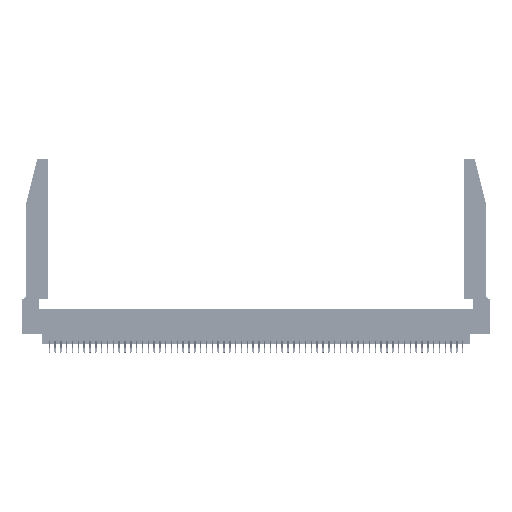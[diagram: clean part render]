
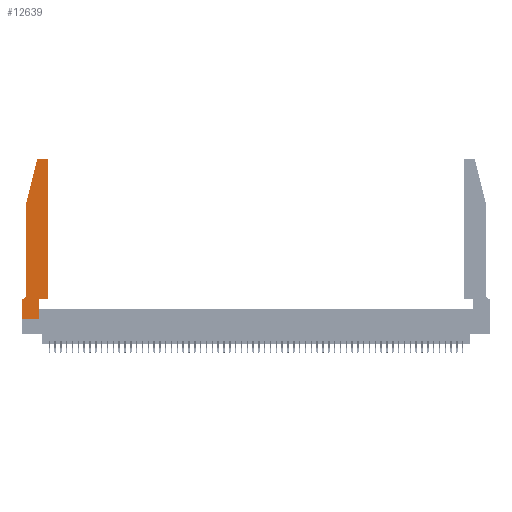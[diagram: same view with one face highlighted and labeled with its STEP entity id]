
A CAD part, top view. The second image highlights one B-rep face of the part: STEP entity #12639.
In plain terms, the highlighted planar face has unit normal (0, 0, 1).
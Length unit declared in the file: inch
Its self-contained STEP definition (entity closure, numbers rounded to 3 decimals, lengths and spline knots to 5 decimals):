
#2148 = CARTESIAN_POINT ( 'NONE',  ( 0.0055, 0.35, 0.37 ) ) ;
#2251 = LINE ( 'NONE', #49824, #40567 ) ;
#2610 = DIRECTION ( 'NONE',  ( -1., 0., 0. ) ) ;
#2852 = VECTOR ( 'NONE', #40689, 39.37008 ) ;
#3091 = ORIENTED_EDGE ( 'NONE', *, *, #7677, .T. ) ;
#3699 = CARTESIAN_POINT ( 'NONE',  ( 0.4505, 2.72, 0.37 ) ) ;
#4174 = CARTESIAN_POINT ( 'NONE',  ( 0.2865, 0., 0.37 ) ) ;
#4948 = EDGE_CURVE ( 'NONE', #49151, #29414, #12987, .T. ) ;
#5057 = CARTESIAN_POINT ( 'NONE',  ( 0., 0., 0.37 ) ) ;
#5948 = CARTESIAN_POINT ( 'NONE',  ( 0.4505, 0.35, 0.37 ) ) ;
#7371 = DIRECTION ( 'NONE',  ( -1., 0., 0. ) ) ;
#7677 = EDGE_CURVE ( 'NONE', #14945, #19600, #40985, .T. ) ;
#8017 = LINE ( 'NONE', #29578, #54001 ) ;
#8201 = LINE ( 'NONE', #17838, #54185 ) ;
#8262 = EDGE_CURVE ( 'NONE', #47192, #46977, #10237, .T. ) ;
#9140 = LINE ( 'NONE', #52116, #30073 ) ;
#9202 = AXIS2_PLACEMENT_3D ( 'NONE', #17067, #48257, #21542 ) ;
#9539 = CARTESIAN_POINT ( 'NONE',  ( 0.4505, 0.35, 0.37 ) ) ;
#9797 = FACE_OUTER_BOUND ( 'NONE', #55685, .T. ) ;
#10224 = VECTOR ( 'NONE', #24977, 39.37008 ) ;
#10237 = LINE ( 'NONE', #5948, #56197 ) ;
#10424 = DIRECTION ( 'NONE',  ( 1., 0., 0. ) ) ;
#12004 = PLANE ( 'NONE',  #14550 ) ;
#12639 = ADVANCED_FACE ( 'NONE', ( #9797 ), #12004, .T. ) ;
#12987 = LINE ( 'NONE', #20457, #10224 ) ;
#14550 = AXIS2_PLACEMENT_3D ( 'NONE', #38724, #43186, #16479 ) ;
#14945 = VERTEX_POINT ( 'NONE', #3699 ) ;
#15173 = EDGE_CURVE ( 'NONE', #46977, #14945, #2251, .T. ) ;
#15523 = EDGE_CURVE ( 'NONE', #15922, #34785, #9140, .T. ) ;
#15922 = VERTEX_POINT ( 'NONE', #54968 ) ;
#16479 = DIRECTION ( 'NONE',  ( 1., 0., 0. ) ) ;
#17067 = CARTESIAN_POINT ( 'NONE',  ( 0.4205, 2.72, 0.37 ) ) ;
#17551 = CARTESIAN_POINT ( 'NONE',  ( 0.0755, 0.42, 0.37 ) ) ;
#17658 = ORIENTED_EDGE ( 'NONE', *, *, #4948, .T. ) ;
#17838 = CARTESIAN_POINT ( 'NONE',  ( 0.2865, 0.35, 0.37 ) ) ;
#18653 = CIRCLE ( 'NONE', #20409, 0.03 ) ;
#19183 = LINE ( 'NONE', #49753, #29698 ) ;
#19394 = EDGE_CURVE ( 'NONE', #30551, #15922, #19183, .T. ) ;
#19600 = VERTEX_POINT ( 'NONE', #55529 ) ;
#19654 = CARTESIAN_POINT ( 'NONE',  ( 0.284, 2.72, 0.37 ) ) ;
#19703 = DIRECTION ( 'NONE',  ( 0., 0., -1. ) ) ;
#20142 = AXIS2_PLACEMENT_3D ( 'NONE', #46410, #19703, #50907 ) ;
#20409 = AXIS2_PLACEMENT_3D ( 'NONE', #19654, #50843, #24186 ) ;
#20457 = CARTESIAN_POINT ( 'NONE',  ( 0., 0., 0.37 ) ) ;
#20567 = CARTESIAN_POINT ( 'NONE',  ( 0.25487, 2.72718, 0.37 ) ) ;
#21542 = DIRECTION ( 'NONE',  ( 1., 0., 0. ) ) ;
#23136 = ORIENTED_EDGE ( 'NONE', *, *, #15523, .T. ) ;
#24186 = DIRECTION ( 'NONE',  ( 1., 0., 0. ) ) ;
#24549 = CIRCLE ( 'NONE', #20142, 0.07 ) ;
#24809 = CARTESIAN_POINT ( 'NONE',  ( 0.2605, 2.75, 0.37 ) ) ;
#24977 = DIRECTION ( 'NONE',  ( 1., 0., 0. ) ) ;
#25826 = EDGE_CURVE ( 'NONE', #28845, #50900, #8017, .T. ) ;
#27555 = DIRECTION ( 'NONE',  ( -0.239, -0.971, 0. ) ) ;
#28845 = VERTEX_POINT ( 'NONE', #2148 ) ;
#29225 = CARTESIAN_POINT ( 'NONE',  ( 0.2865, 0.35, 0.37 ) ) ;
#29333 = LINE ( 'NONE', #5057, #2852 ) ;
#29414 = VERTEX_POINT ( 'NONE', #4174 ) ;
#29578 = CARTESIAN_POINT ( 'NONE',  ( 0.0755, 0.35, 0.37 ) ) ;
#29698 = VECTOR ( 'NONE', #27555, 39.37008 ) ;
#30073 = VECTOR ( 'NONE', #47618, 39.37008 ) ;
#30551 = VERTEX_POINT ( 'NONE', #20567 ) ;
#30716 = CARTESIAN_POINT ( 'NONE',  ( 0., 0.35, 0.37 ) ) ;
#32956 = ORIENTED_EDGE ( 'NONE', *, *, #37030, .T. ) ;
#33186 = EDGE_CURVE ( 'NONE', #39504, #30551, #18653, .T. ) ;
#33456 = ORIENTED_EDGE ( 'NONE', *, *, #25826, .T. ) ;
#33618 = EDGE_CURVE ( 'NONE', #29414, #47192, #8201, .T. ) ;
#33812 = CARTESIAN_POINT ( 'NONE',  ( 0.284, 2.75, 0.37 ) ) ;
#34785 = VERTEX_POINT ( 'NONE', #17551 ) ;
#34928 = ORIENTED_EDGE ( 'NONE', *, *, #19394, .T. ) ;
#35371 = EDGE_CURVE ( 'NONE', #19600, #39504, #49142, .T. ) ;
#35889 = VECTOR ( 'NONE', #2610, 39.37008 ) ;
#36342 = ORIENTED_EDGE ( 'NONE', *, *, #33618, .T. ) ;
#37030 = EDGE_CURVE ( 'NONE', #34785, #28845, #24549, .T. ) ;
#38724 = CARTESIAN_POINT ( 'NONE',  ( 0., 0.35, 0.37 ) ) ;
#39504 = VERTEX_POINT ( 'NONE', #33812 ) ;
#39659 = ORIENTED_EDGE ( 'NONE', *, *, #35371, .T. ) ;
#40567 = VECTOR ( 'NONE', #54284, 39.37008 ) ;
#40689 = DIRECTION ( 'NONE',  ( 0., -1., 0. ) ) ;
#40985 = CIRCLE ( 'NONE', #9202, 0.03 ) ;
#41093 = DIRECTION ( 'NONE',  ( 0., 1., 0. ) ) ;
#43186 = DIRECTION ( 'NONE',  ( 0., 0., 1. ) ) ;
#45943 = ORIENTED_EDGE ( 'NONE', *, *, #33186, .T. ) ;
#46410 = CARTESIAN_POINT ( 'NONE',  ( 0.0055, 0.42, 0.37 ) ) ;
#46977 = VERTEX_POINT ( 'NONE', #9539 ) ;
#47192 = VERTEX_POINT ( 'NONE', #29225 ) ;
#47618 = DIRECTION ( 'NONE',  ( 0., -1., 0. ) ) ;
#48197 = ORIENTED_EDGE ( 'NONE', *, *, #8262, .T. ) ;
#48257 = DIRECTION ( 'NONE',  ( 0., 0., 1. ) ) ;
#49142 = LINE ( 'NONE', #24809, #35889 ) ;
#49151 = VERTEX_POINT ( 'NONE', #56822 ) ;
#49753 = CARTESIAN_POINT ( 'NONE',  ( 0.0755, 2., 0.37 ) ) ;
#49824 = CARTESIAN_POINT ( 'NONE',  ( 0.4505, 0.35, 0.37 ) ) ;
#50379 = EDGE_CURVE ( 'NONE', #50900, #49151, #29333, .T. ) ;
#50843 = DIRECTION ( 'NONE',  ( 0., 0., 1. ) ) ;
#50900 = VERTEX_POINT ( 'NONE', #30716 ) ;
#50907 = DIRECTION ( 'NONE',  ( -1., 0., 0. ) ) ;
#52116 = CARTESIAN_POINT ( 'NONE',  ( 0.0755, 2., 0.37 ) ) ;
#52131 = ORIENTED_EDGE ( 'NONE', *, *, #50379, .T. ) ;
#53178 = ORIENTED_EDGE ( 'NONE', *, *, #15173, .T. ) ;
#54001 = VECTOR ( 'NONE', #7371, 39.37008 ) ;
#54185 = VECTOR ( 'NONE', #41093, 39.37008 ) ;
#54284 = DIRECTION ( 'NONE',  ( 0., 1., 0. ) ) ;
#54968 = CARTESIAN_POINT ( 'NONE',  ( 0.0755, 2., 0.37 ) ) ;
#55529 = CARTESIAN_POINT ( 'NONE',  ( 0.4205, 2.75, 0.37 ) ) ;
#55685 = EDGE_LOOP ( 'NONE', ( #39659, #45943, #34928, #23136, #32956, #33456, #52131, #17658, #36342, #48197, #53178, #3091 ) ) ;
#56197 = VECTOR ( 'NONE', #10424, 39.37008 ) ;
#56822 = CARTESIAN_POINT ( 'NONE',  ( 0., 0., 0.37 ) ) ;
